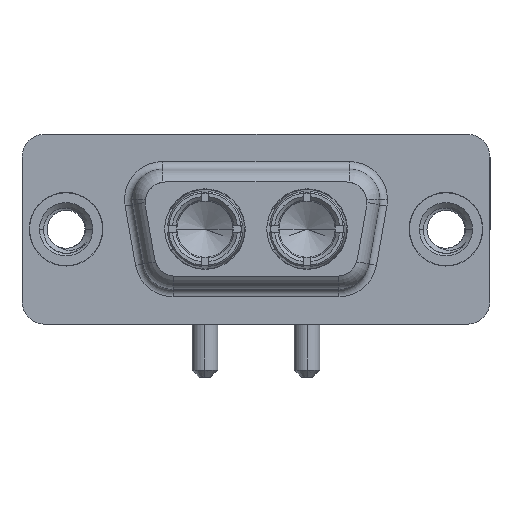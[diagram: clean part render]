
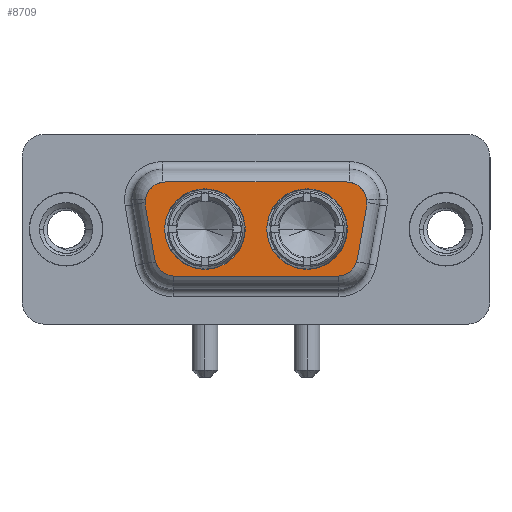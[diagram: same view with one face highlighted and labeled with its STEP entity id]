
A CAD part, top view. The second image highlights one B-rep face of the part: STEP entity #8709.
In plain terms, the highlighted planar face has unit normal (0, 0, 1).
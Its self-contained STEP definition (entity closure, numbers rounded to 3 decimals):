
#95 = CARTESIAN_POINT ( 'NONE',  ( 5.838, -1.984, 6.2 ) ) ;
#234 = CARTESIAN_POINT ( 'NONE',  ( 19.779, 1.516, 6.2 ) ) ;
#276 = ORIENTED_EDGE ( 'NONE', *, *, #3787, .T. ) ;
#338 = AXIS2_PLACEMENT_3D ( 'NONE', #6882, #10499, #9575 ) ;
#348 = VERTEX_POINT ( 'NONE', #7917 ) ;
#468 = CARTESIAN_POINT ( 'NONE',  ( 7.167, -3.1, 6.2 ) ) ;
#540 = DIRECTION ( 'NONE',  ( -1., 0., 0. ) ) ;
#696 = DIRECTION ( 'NONE',  ( -1., 0., 0. ) ) ;
#778 = FACE_BOUND ( 'NONE', #3405, .T. ) ;
#916 = DIRECTION ( 'NONE',  ( 0., 0., 1. ) ) ;
#921 = VERTEX_POINT ( 'NONE', #2203 ) ;
#1078 = DIRECTION ( 'NONE',  ( 0.174, -0.985, 0. ) ) ;
#1176 = DIRECTION ( 'NONE',  ( 0.174, 0.985, 0. ) ) ;
#1603 = CIRCLE ( 'NONE', #6112, 1.35 ) ;
#1716 = DIRECTION ( 'NONE',  ( 1., 0., 0. ) ) ;
#1761 = DIRECTION ( 'NONE',  ( 0., 0., -1. ) ) ;
#1797 = CIRCLE ( 'NONE', #6106, 1.35 ) ;
#1958 = DIRECTION ( 'NONE',  ( -1., 0., 0. ) ) ;
#2025 = CARTESIAN_POINT ( 'NONE',  ( 17.833, -3.1, 6.2 ) ) ;
#2203 = CARTESIAN_POINT ( 'NONE',  ( 5.838, -1.984, 6.2 ) ) ;
#2218 = EDGE_CURVE ( 'NONE', #921, #8062, #7617, .T. ) ;
#2338 = AXIS2_PLACEMENT_3D ( 'NONE', #9321, #916, #1958 ) ;
#2559 = CARTESIAN_POINT ( 'NONE',  ( 13.21, 0., 6.2 ) ) ;
#2717 = CARTESIAN_POINT ( 'NONE',  ( 17.833, -1.75, 6.2 ) ) ;
#3405 = EDGE_LOOP ( 'NONE', ( #4400, #7164 ) ) ;
#3562 = AXIS2_PLACEMENT_3D ( 'NONE', #10379, #6528, #4871 ) ;
#3727 = DIRECTION ( 'NONE',  ( 1., 0., 0. ) ) ;
#3731 = VERTEX_POINT ( 'NONE', #7696 ) ;
#3787 = EDGE_CURVE ( 'NONE', #348, #8195, #1797, .T. ) ;
#3862 = AXIS2_PLACEMENT_3D ( 'NONE', #8279, #4601, #1716 ) ;
#3889 = DIRECTION ( 'NONE',  ( 0., 0., 1. ) ) ;
#3899 = VERTEX_POINT ( 'NONE', #11288 ) ;
#3950 = DIRECTION ( 'NONE',  ( 1., 0., 0. ) ) ;
#3965 = CIRCLE ( 'NONE', #6908, 2.65 ) ;
#4059 = AXIS2_PLACEMENT_3D ( 'NONE', #7293, #11045, #9261 ) ;
#4147 = VERTEX_POINT ( 'NONE', #234 ) ;
#4198 = ORIENTED_EDGE ( 'NONE', *, *, #12053, .F. ) ;
#4258 = ORIENTED_EDGE ( 'NONE', *, *, #2218, .T. ) ;
#4270 = EDGE_CURVE ( 'NONE', #4147, #5248, #1603, .T. ) ;
#4400 = ORIENTED_EDGE ( 'NONE', *, *, #5384, .F. ) ;
#4452 = PLANE ( 'NONE',  #8351 ) ;
#4566 = AXIS2_PLACEMENT_3D ( 'NONE', #2717, #7188, #696 ) ;
#4601 = DIRECTION ( 'NONE',  ( 0., 0., 1. ) ) ;
#4681 = CARTESIAN_POINT ( 'NONE',  ( 9.14, 0., 6.2 ) ) ;
#4737 = VECTOR ( 'NONE', #1176, 1000. ) ;
#4827 = VERTEX_POINT ( 'NONE', #2559 ) ;
#4871 = DIRECTION ( 'NONE',  ( 1., 0., 0. ) ) ;
#5023 = VECTOR ( 'NONE', #1078, 1000. ) ;
#5089 = EDGE_CURVE ( 'NONE', #6286, #7505, #11030, .T. ) ;
#5211 = DIRECTION ( 'NONE',  ( 0., 0., 1. ) ) ;
#5242 = EDGE_LOOP ( 'NONE', ( #4258, #8832, #11706, #11727, #9137, #11875, #6300, #276, #7024 ) ) ;
#5248 = VERTEX_POINT ( 'NONE', #5661 ) ;
#5384 = EDGE_CURVE ( 'NONE', #3731, #3899, #3965, .T. ) ;
#5488 = EDGE_LOOP ( 'NONE', ( #8058, #4198 ) ) ;
#5511 = CARTESIAN_POINT ( 'NONE',  ( 19.162, -1.984, 6.2 ) ) ;
#5661 = CARTESIAN_POINT ( 'NONE',  ( 18.45, 3.1, 6.2 ) ) ;
#5834 = EDGE_CURVE ( 'NONE', #7505, #4147, #11305, .T. ) ;
#6106 = AXIS2_PLACEMENT_3D ( 'NONE', #10518, #3889, #3950 ) ;
#6112 = AXIS2_PLACEMENT_3D ( 'NONE', #8021, #5211, #540 ) ;
#6286 = VERTEX_POINT ( 'NONE', #2025 ) ;
#6300 = ORIENTED_EDGE ( 'NONE', *, *, #10010, .T. ) ;
#6528 = DIRECTION ( 'NONE',  ( 0., 0., 1. ) ) ;
#6577 = DIRECTION ( 'NONE',  ( 1., 0., 0. ) ) ;
#6608 = LINE ( 'NONE', #10343, #6923 ) ;
#6882 = CARTESIAN_POINT ( 'NONE',  ( 9.14, 0., 6.2 ) ) ;
#6908 = AXIS2_PLACEMENT_3D ( 'NONE', #4681, #7496, #6577 ) ;
#6923 = VECTOR ( 'NONE', #7894, 1000. ) ;
#7024 = ORIENTED_EDGE ( 'NONE', *, *, #10909, .T. ) ;
#7164 = ORIENTED_EDGE ( 'NONE', *, *, #9500, .F. ) ;
#7188 = DIRECTION ( 'NONE',  ( 0., 0., 1. ) ) ;
#7293 = CARTESIAN_POINT ( 'NONE',  ( 15.86, 0., 6.2 ) ) ;
#7338 = FACE_OUTER_BOUND ( 'NONE', #5242, .T. ) ;
#7345 = CARTESIAN_POINT ( 'NONE',  ( 17.833, -3.1, 6.2 ) ) ;
#7407 = CARTESIAN_POINT ( 'NONE',  ( 5.221, 1.516, 6.2 ) ) ;
#7468 = EDGE_CURVE ( 'NONE', #8062, #6286, #9248, .T. ) ;
#7496 = DIRECTION ( 'NONE',  ( 0., 0., 1. ) ) ;
#7505 = VERTEX_POINT ( 'NONE', #5511 ) ;
#7617 = CIRCLE ( 'NONE', #2338, 1.35 ) ;
#7696 = CARTESIAN_POINT ( 'NONE',  ( 11.79, 0., 6.2 ) ) ;
#7894 = DIRECTION ( 'NONE',  ( -1., 0., 0. ) ) ;
#7917 = CARTESIAN_POINT ( 'NONE',  ( 5.2, 1.75, 6.2 ) ) ;
#7922 = EDGE_CURVE ( 'NONE', #5248, #9362, #6608, .T. ) ;
#8021 = CARTESIAN_POINT ( 'NONE',  ( 18.45, 1.75, 6.2 ) ) ;
#8058 = ORIENTED_EDGE ( 'NONE', *, *, #12134, .F. ) ;
#8062 = VERTEX_POINT ( 'NONE', #468 ) ;
#8194 = CARTESIAN_POINT ( 'NONE',  ( 7.167, -1.75, 6.2 ) ) ;
#8195 = VERTEX_POINT ( 'NONE', #7407 ) ;
#8246 = VERTEX_POINT ( 'NONE', #11835 ) ;
#8258 = DIRECTION ( 'NONE',  ( -1., 0., 0. ) ) ;
#8279 = CARTESIAN_POINT ( 'NONE',  ( 15.86, 0., 6.2 ) ) ;
#8351 = AXIS2_PLACEMENT_3D ( 'NONE', #8194, #1761, #8258 ) ;
#8709 = ADVANCED_FACE ( 'NONE', ( #10153, #778, #7338 ), #4452, .F. ) ;
#8832 = ORIENTED_EDGE ( 'NONE', *, *, #7468, .T. ) ;
#8840 = CIRCLE ( 'NONE', #3562, 1.35 ) ;
#9137 = ORIENTED_EDGE ( 'NONE', *, *, #4270, .T. ) ;
#9146 = CIRCLE ( 'NONE', #338, 2.65 ) ;
#9248 = LINE ( 'NONE', #7345, #10432 ) ;
#9261 = DIRECTION ( 'NONE',  ( 1., 0., 0. ) ) ;
#9321 = CARTESIAN_POINT ( 'NONE',  ( 7.167, -1.75, 6.2 ) ) ;
#9362 = VERTEX_POINT ( 'NONE', #9699 ) ;
#9368 = CIRCLE ( 'NONE', #3862, 2.65 ) ;
#9480 = LINE ( 'NONE', #95, #5023 ) ;
#9500 = EDGE_CURVE ( 'NONE', #3899, #3731, #9146, .T. ) ;
#9573 = CARTESIAN_POINT ( 'NONE',  ( 19.779, 1.516, 6.2 ) ) ;
#9575 = DIRECTION ( 'NONE',  ( 1., 0., 0. ) ) ;
#9699 = CARTESIAN_POINT ( 'NONE',  ( 6.55, 3.1, 6.2 ) ) ;
#10010 = EDGE_CURVE ( 'NONE', #9362, #348, #8840, .T. ) ;
#10153 = FACE_BOUND ( 'NONE', #5488, .T. ) ;
#10343 = CARTESIAN_POINT ( 'NONE',  ( 6.55, 3.1, 6.2 ) ) ;
#10379 = CARTESIAN_POINT ( 'NONE',  ( 6.55, 1.75, 6.2 ) ) ;
#10432 = VECTOR ( 'NONE', #3727, 1000. ) ;
#10499 = DIRECTION ( 'NONE',  ( 0., 0., 1. ) ) ;
#10518 = CARTESIAN_POINT ( 'NONE',  ( 6.55, 1.75, 6.2 ) ) ;
#10732 = CIRCLE ( 'NONE', #4059, 2.65 ) ;
#10909 = EDGE_CURVE ( 'NONE', #8195, #921, #9480, .T. ) ;
#11030 = CIRCLE ( 'NONE', #4566, 1.35 ) ;
#11045 = DIRECTION ( 'NONE',  ( 0., 0., 1. ) ) ;
#11288 = CARTESIAN_POINT ( 'NONE',  ( 6.49, 0., 6.2 ) ) ;
#11305 = LINE ( 'NONE', #9573, #4737 ) ;
#11706 = ORIENTED_EDGE ( 'NONE', *, *, #5089, .T. ) ;
#11727 = ORIENTED_EDGE ( 'NONE', *, *, #5834, .T. ) ;
#11835 = CARTESIAN_POINT ( 'NONE',  ( 18.51, 0., 6.2 ) ) ;
#11875 = ORIENTED_EDGE ( 'NONE', *, *, #7922, .T. ) ;
#12053 = EDGE_CURVE ( 'NONE', #4827, #8246, #9368, .T. ) ;
#12134 = EDGE_CURVE ( 'NONE', #8246, #4827, #10732, .T. ) ;
